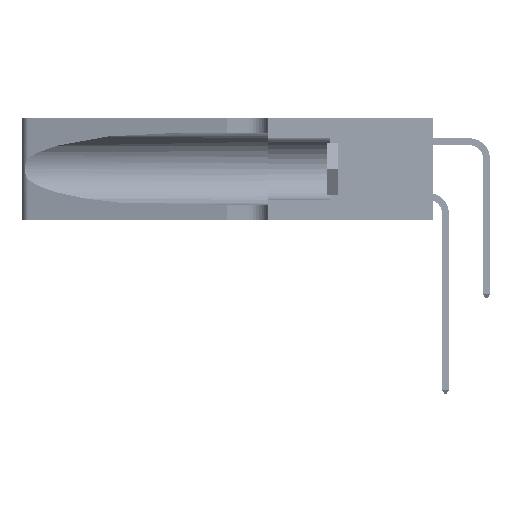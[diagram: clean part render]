
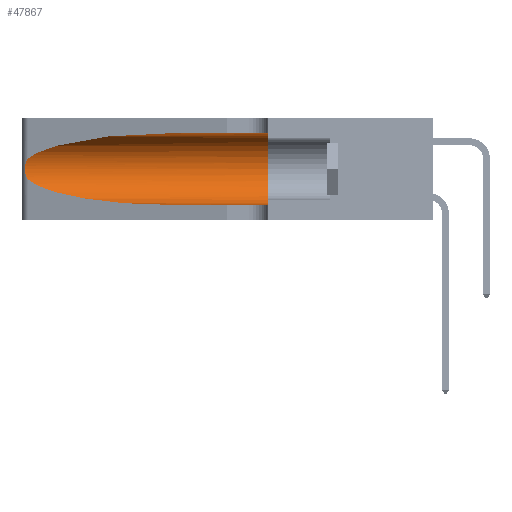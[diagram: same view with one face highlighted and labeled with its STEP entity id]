
A CAD part, left-side view. The second image highlights one B-rep face of the part: STEP entity #47867.
In plain terms, the highlighted cylindrical face has radius 3.308 mm (diameter 6.617 mm), a partial arc.
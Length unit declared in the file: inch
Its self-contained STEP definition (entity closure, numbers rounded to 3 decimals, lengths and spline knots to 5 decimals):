
#88 = VERTEX_POINT ( 'NONE', #26576 ) ;
#416 = CARTESIAN_POINT ( 'NONE',  ( 0.1305, 1.61858, 0.31525 ) ) ;
#1740 = CARTESIAN_POINT ( 'NONE',  ( 0.25487, 1.22718, 0.14631 ) ) ;
#2230 = CARTESIAN_POINT ( 'NONE',  ( 0.18966, 0.96281, 0.31525 ) ) ;
#2389 = CARTESIAN_POINT ( 'NONE',  ( 0.25487, 1.22718, 0.22369 ) ) ;
#3087 = CARTESIAN_POINT ( 'NONE',  ( 0.25487, 1.22718, 0.14631 ) ) ;
#3771 = DIRECTION ( 'NONE',  ( 0., 0., -1. ) ) ;
#4858 = DIRECTION ( 'NONE',  ( 0., 1., 0. ) ) ;
#4961 =( BOUNDED_CURVE ( )  B_SPLINE_CURVE ( 3, ( #9850, #2230, #25139, #2389 ),
 .UNSPECIFIED., .F., .T. ) 
 B_SPLINE_CURVE_WITH_KNOTS ( ( 4, 4 ),
 ( 1.5708, 2.84003 ),
 .UNSPECIFIED. ) 
 CURVE ( )  GEOMETRIC_REPRESENTATION_ITEM ( )  RATIONAL_B_SPLINE_CURVE ( ( 1., 0.87, 0.87, 1. ) ) 
 REPRESENTATION_ITEM ( '' )  );
#5777 = ORIENTED_EDGE ( 'NONE', *, *, #22535, .F. ) ;
#6648 = VECTOR ( 'NONE', #34627, 39.37008 ) ;
#6731 = CARTESIAN_POINT ( 'NONE',  ( 0.25639, 1.23184, 0.21858 ) ) ;
#7565 = DIRECTION ( 'NONE',  ( 0., -1., 0. ) ) ;
#9356 = CARTESIAN_POINT ( 'NONE',  ( 0.1305, 0.72297, 0.05475 ) ) ;
#9850 = CARTESIAN_POINT ( 'NONE',  ( 0.1305, 0.72297, 0.31525 ) ) ;
#10583 = CARTESIAN_POINT ( 'NONE',  ( 0.25854, 1.2359, 0.20912 ) ) ;
#12210 = LINE ( 'NONE', #18107, #42480 ) ;
#12841 = VERTEX_POINT ( 'NONE', #14386 ) ;
#12885 = ORIENTED_EDGE ( 'NONE', *, *, #32687, .T. ) ;
#13255 = AXIS2_PLACEMENT_3D ( 'NONE', #30350, #7565, #3771 ) ;
#13386 = EDGE_CURVE ( 'NONE', #88, #19128, #4961, .T. ) ;
#14215 = CARTESIAN_POINT ( 'NONE',  ( 0.25487, 1.22718, 0.22369 ) ) ;
#14375 = CARTESIAN_POINT ( 'NONE',  ( 0.26075, 1.23896, 0.19203 ) ) ;
#14386 = CARTESIAN_POINT ( 'NONE',  ( 0.25487, 1.22718, 0.14631 ) ) ;
#14938 = EDGE_CURVE ( 'NONE', #12841, #40697, #36610, .T. ) ;
#16290 = VERTEX_POINT ( 'NONE', #24687 ) ;
#18107 = CARTESIAN_POINT ( 'NONE',  ( 0.1305, 1.61858, 0.05475 ) ) ;
#18174 = CARTESIAN_POINT ( 'NONE',  ( 0.26017, 1.23833, 0.17102 ) ) ;
#18540 = VERTEX_POINT ( 'NONE', #35298 ) ;
#19128 = VERTEX_POINT ( 'NONE', #27958 ) ;
#21265 = ORIENTED_EDGE ( 'NONE', *, *, #24954, .F. ) ;
#22044 = CARTESIAN_POINT ( 'NONE',  ( 0.25789, 1.23486, 0.15765 ) ) ;
#22106 = AXIS2_PLACEMENT_3D ( 'NONE', #27612, #4858, #31445 ) ;
#22535 = EDGE_CURVE ( 'NONE', #88, #18540, #35769, .T. ) ;
#22622 = CIRCLE ( 'NONE', #22106, 0.13025 ) ;
#22730 = ORIENTED_EDGE ( 'NONE', *, *, #14938, .T. ) ;
#24483 = CARTESIAN_POINT ( 'NONE',  ( 0.2373, 1.15595, 0.08982 ) ) ;
#24687 = CARTESIAN_POINT ( 'NONE',  ( 0.1305, 0.35, 0.05475 ) ) ;
#24954 = EDGE_CURVE ( 'NONE', #18540, #16290, #22622, .T. ) ;
#25139 = CARTESIAN_POINT ( 'NONE',  ( 0.2373, 1.15595, 0.28018 ) ) ;
#25851 = CARTESIAN_POINT ( 'NONE',  ( 0.25555, 1.22993, 0.14849 ) ) ;
#26576 = CARTESIAN_POINT ( 'NONE',  ( 0.1305, 0.72297, 0.31525 ) ) ;
#27612 = CARTESIAN_POINT ( 'NONE',  ( 0.1305, 0.35, 0.185 ) ) ;
#27958 = CARTESIAN_POINT ( 'NONE',  ( 0.25487, 1.22718, 0.22369 ) ) ;
#28970 = CARTESIAN_POINT ( 'NONE',  ( 0.1305, 0.72297, 0.05475 ) ) ;
#30350 = CARTESIAN_POINT ( 'NONE',  ( 0.1305, 1.61858, 0.185 ) ) ;
#31445 = DIRECTION ( 'NONE',  ( 0., 0., 1. ) ) ;
#32111 = CARTESIAN_POINT ( 'NONE',  ( 0.18966, 0.96281, 0.05475 ) ) ;
#32687 = EDGE_CURVE ( 'NONE', #40697, #16290, #12210, .T. ) ;
#32864 = CYLINDRICAL_SURFACE ( 'NONE', #13255, 0.13025 ) ;
#33305 = CARTESIAN_POINT ( 'NONE',  ( 0.25787, 1.23484, 0.2124 ) ) ;
#33734 = ORIENTED_EDGE ( 'NONE', *, *, #13386, .T. ) ;
#34627 = DIRECTION ( 'NONE',  ( 0., -1., 0. ) ) ;
#35298 = CARTESIAN_POINT ( 'NONE',  ( 0.1305, 0.35, 0.31525 ) ) ;
#35769 = LINE ( 'NONE', #416, #6648 ) ;
#36610 =( BOUNDED_CURVE ( )  B_SPLINE_CURVE ( 3, ( #1740, #24483, #32111, #9356 ),
 .UNSPECIFIED., .F., .F. ) 
 B_SPLINE_CURVE_WITH_KNOTS ( ( 4, 4 ),
 ( 3.44316, 4.71239 ),
 .UNSPECIFIED. ) 
 CURVE ( )  GEOMETRIC_REPRESENTATION_ITEM ( )  RATIONAL_B_SPLINE_CURVE ( ( 1., 0.87, 0.87, 1. ) ) 
 REPRESENTATION_ITEM ( '' )  );
#36969 = CARTESIAN_POINT ( 'NONE',  ( 0.25555, 1.22994, 0.2215 ) ) ;
#37125 = CARTESIAN_POINT ( 'NONE',  ( 0.26018, 1.23835, 0.19895 ) ) ;
#38134 = B_SPLINE_CURVE_WITH_KNOTS ( 'NONE', 3,
 ( #14215, #36969, #6731, #33305, #10583, #37125, #14375, #40956, #18174, #44723, #22044, #48531, #25851, #3087 ),
 .UNSPECIFIED., .F., .F.,
 ( 4, 2, 2, 2, 2, 2, 4 ),
 ( 0., 0.00027, 0.00053, 0.00107, 0.0016, 0.00187, 0.00214 ),
 .UNSPECIFIED. ) ;
#40697 = VERTEX_POINT ( 'NONE', #28970 ) ;
#40956 = CARTESIAN_POINT ( 'NONE',  ( 0.26075, 1.23896, 0.178 ) ) ;
#42480 = VECTOR ( 'NONE', #48456, 39.37008 ) ;
#42921 = EDGE_LOOP ( 'NONE', ( #33734, #44561, #22730, #12885, #21265, #5777 ) ) ;
#44121 = FACE_OUTER_BOUND ( 'NONE', #42921, .T. ) ;
#44561 = ORIENTED_EDGE ( 'NONE', *, *, #46984, .T. ) ;
#44723 = CARTESIAN_POINT ( 'NONE',  ( 0.25856, 1.23593, 0.16098 ) ) ;
#46984 = EDGE_CURVE ( 'NONE', #19128, #12841, #38134, .T. ) ;
#47867 = ADVANCED_FACE ( 'NONE', ( #44121 ), #32864, .F. ) ;
#48456 = DIRECTION ( 'NONE',  ( 0., -1., 0. ) ) ;
#48531 = CARTESIAN_POINT ( 'NONE',  ( 0.25639, 1.23186, 0.15144 ) ) ;
